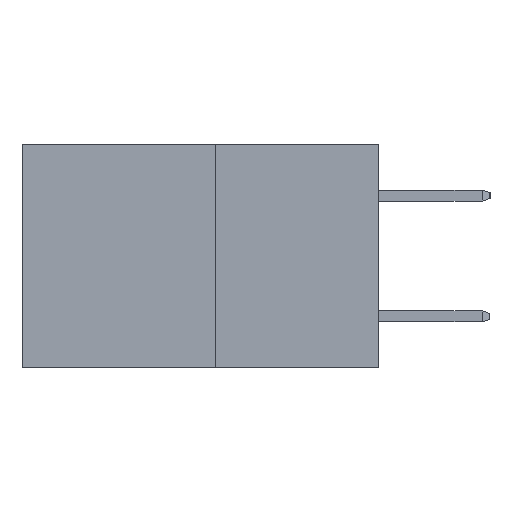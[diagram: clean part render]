
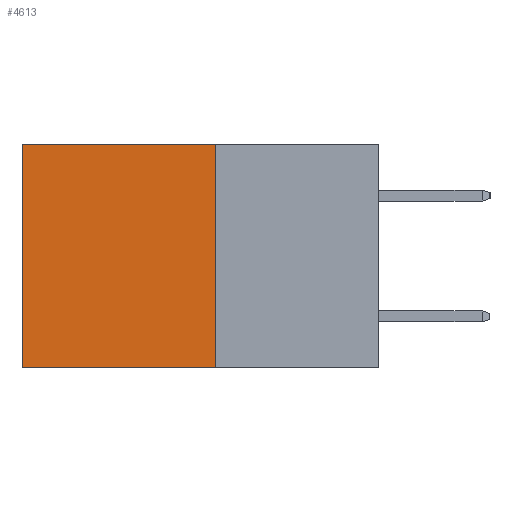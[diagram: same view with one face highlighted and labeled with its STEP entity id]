
A CAD part, left-side view. The second image highlights one B-rep face of the part: STEP entity #4613.
In plain terms, the highlighted planar face has unit normal (-1, 0, 0).
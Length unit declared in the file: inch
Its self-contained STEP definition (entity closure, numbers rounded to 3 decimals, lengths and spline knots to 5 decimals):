
#86 = EDGE_CURVE ( 'NONE', #5521, #707, #7208, .T. ) ;
#289 = AXIS2_PLACEMENT_3D ( 'NONE', #1684, #1643, #1631 ) ;
#707 = VERTEX_POINT ( 'NONE', #859 ) ;
#784 = EDGE_CURVE ( 'NONE', #5670, #5521, #1433, .T. ) ;
#859 = CARTESIAN_POINT ( 'NONE',  ( 0.277, 0.59, -0.37 ) ) ;
#911 = CARTESIAN_POINT ( 'NONE',  ( 0.277, 0.27, -0.37 ) ) ;
#999 = DIRECTION ( 'NONE',  ( 0., 1., 0. ) ) ;
#1104 = CARTESIAN_POINT ( 'NONE',  ( 0.277, 0.27, 0. ) ) ;
#1261 = CARTESIAN_POINT ( 'NONE',  ( 0.277, 0.59, -0.37 ) ) ;
#1433 = LINE ( 'NONE', #911, #11154 ) ;
#1631 = DIRECTION ( 'NONE',  ( 0., 0., -1. ) ) ;
#1643 = DIRECTION ( 'NONE',  ( 1., 0., 0. ) ) ;
#1684 = CARTESIAN_POINT ( 'NONE',  ( 0.277, 0.27, -0.37 ) ) ;
#1709 = PLANE ( 'NONE',  #289 ) ;
#1855 = VECTOR ( 'NONE', #4194, 39.37008 ) ;
#4150 = EDGE_LOOP ( 'NONE', ( #6837, #6359, #6317, #5318 ) ) ;
#4194 = DIRECTION ( 'NONE',  ( 0., 0., -1. ) ) ;
#4415 = LINE ( 'NONE', #1261, #1855 ) ;
#4613 = ADVANCED_FACE ( 'NONE', ( #11613 ), #1709, .F. ) ;
#4669 = EDGE_CURVE ( 'NONE', #5670, #7812, #11351, .T. ) ;
#5318 = ORIENTED_EDGE ( 'NONE', *, *, #4669, .T. ) ;
#5521 = VERTEX_POINT ( 'NONE', #6669 ) ;
#5670 = VERTEX_POINT ( 'NONE', #8786 ) ;
#5721 = CARTESIAN_POINT ( 'NONE',  ( 0.277, 0.27, -0.37 ) ) ;
#6317 = ORIENTED_EDGE ( 'NONE', *, *, #784, .F. ) ;
#6359 = ORIENTED_EDGE ( 'NONE', *, *, #86, .F. ) ;
#6669 = CARTESIAN_POINT ( 'NONE',  ( 0.277, 0.27, -0.37 ) ) ;
#6837 = ORIENTED_EDGE ( 'NONE', *, *, #9431, .T. ) ;
#7208 = LINE ( 'NONE', #5721, #11855 ) ;
#7445 = DIRECTION ( 'NONE',  ( 0., 1., 0. ) ) ;
#7812 = VERTEX_POINT ( 'NONE', #9049 ) ;
#7818 = DIRECTION ( 'NONE',  ( 0., 0., -1. ) ) ;
#8579 = VECTOR ( 'NONE', #999, 39.37008 ) ;
#8786 = CARTESIAN_POINT ( 'NONE',  ( 0.277, 0.27, 0. ) ) ;
#9049 = CARTESIAN_POINT ( 'NONE',  ( 0.277, 0.59, 0. ) ) ;
#9431 = EDGE_CURVE ( 'NONE', #7812, #707, #4415, .T. ) ;
#11154 = VECTOR ( 'NONE', #7818, 39.37008 ) ;
#11351 = LINE ( 'NONE', #1104, #8579 ) ;
#11613 = FACE_OUTER_BOUND ( 'NONE', #4150, .T. ) ;
#11855 = VECTOR ( 'NONE', #7445, 39.37008 ) ;
